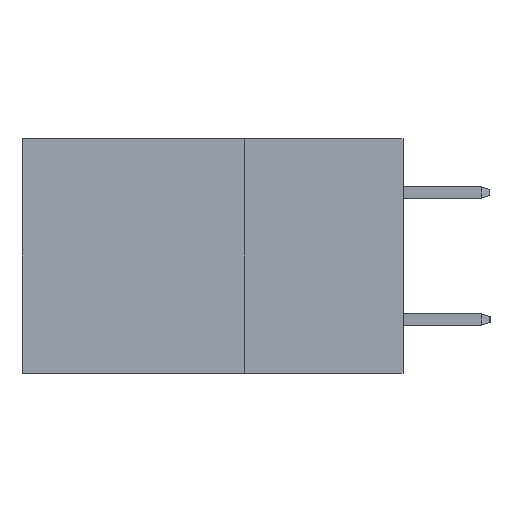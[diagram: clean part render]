
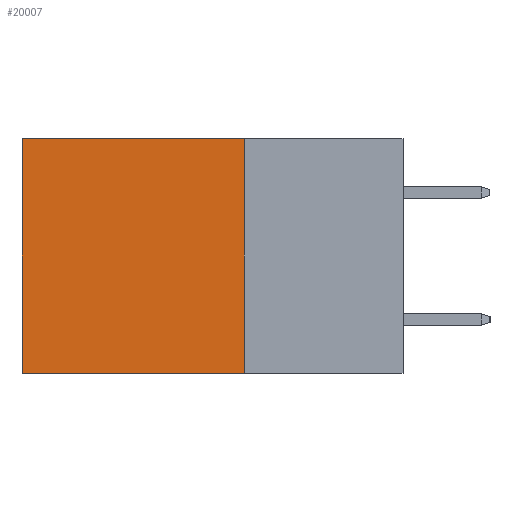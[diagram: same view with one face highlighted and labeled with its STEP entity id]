
A CAD part, left-side view. The second image highlights one B-rep face of the part: STEP entity #20007.
In plain terms, the highlighted planar face has unit normal (-1, 0, 0).
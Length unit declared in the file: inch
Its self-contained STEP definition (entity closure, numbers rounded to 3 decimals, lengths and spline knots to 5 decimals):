
#1389 = ORIENTED_EDGE ( 'NONE', *, *, #18552, .T. ) ;
#2370 = VECTOR ( 'NONE', #10295, 39.37008 ) ;
#5081 = CARTESIAN_POINT ( 'NONE',  ( 0.2875, 0.25, 0. ) ) ;
#5689 = VECTOR ( 'NONE', #16254, 39.37008 ) ;
#5801 = CARTESIAN_POINT ( 'NONE',  ( 0.2875, 0.6, -0.37 ) ) ;
#6368 = VERTEX_POINT ( 'NONE', #16422 ) ;
#6404 = ORIENTED_EDGE ( 'NONE', *, *, #15718, .F. ) ;
#7039 = VECTOR ( 'NONE', #16018, 39.37008 ) ;
#7768 = CARTESIAN_POINT ( 'NONE',  ( 0.2875, 0.25, 0. ) ) ;
#8070 = VERTEX_POINT ( 'NONE', #12647 ) ;
#8123 = PLANE ( 'NONE',  #14566 ) ;
#8311 = CARTESIAN_POINT ( 'NONE',  ( 0.2875, 0.25, -0.37 ) ) ;
#8497 = LINE ( 'NONE', #16744, #8843 ) ;
#8843 = VECTOR ( 'NONE', #18199, 39.37008 ) ;
#9466 = ORIENTED_EDGE ( 'NONE', *, *, #10419, .T. ) ;
#10295 = DIRECTION ( 'NONE',  ( 0., 1., 0. ) ) ;
#10419 = EDGE_CURVE ( 'NONE', #8070, #10884, #11561, .T. ) ;
#10424 = EDGE_CURVE ( 'NONE', #17160, #10884, #13322, .T. ) ;
#10884 = VERTEX_POINT ( 'NONE', #5801 ) ;
#11474 = DIRECTION ( 'NONE',  ( 0., 0., -1. ) ) ;
#11561 = LINE ( 'NONE', #19651, #5689 ) ;
#12615 = FACE_OUTER_BOUND ( 'NONE', #17420, .T. ) ;
#12647 = CARTESIAN_POINT ( 'NONE',  ( 0.2875, 0.6, 0. ) ) ;
#13322 = LINE ( 'NONE', #8311, #2370 ) ;
#13399 = CARTESIAN_POINT ( 'NONE',  ( 0.2875, 0.25, -0.37 ) ) ;
#14237 = LINE ( 'NONE', #7768, #7039 ) ;
#14566 = AXIS2_PLACEMENT_3D ( 'NONE', #5081, #19069, #11474 ) ;
#15238 = ORIENTED_EDGE ( 'NONE', *, *, #10424, .F. ) ;
#15718 = EDGE_CURVE ( 'NONE', #6368, #17160, #14237, .T. ) ;
#16018 = DIRECTION ( 'NONE',  ( 0., 0., -1. ) ) ;
#16254 = DIRECTION ( 'NONE',  ( 0., 0., -1. ) ) ;
#16422 = CARTESIAN_POINT ( 'NONE',  ( 0.2875, 0.25, 0. ) ) ;
#16744 = CARTESIAN_POINT ( 'NONE',  ( 0.2875, 0.25, 0. ) ) ;
#17160 = VERTEX_POINT ( 'NONE', #13399 ) ;
#17420 = EDGE_LOOP ( 'NONE', ( #9466, #15238, #6404, #1389 ) ) ;
#18199 = DIRECTION ( 'NONE',  ( 0., 1., 0. ) ) ;
#18552 = EDGE_CURVE ( 'NONE', #6368, #8070, #8497, .T. ) ;
#19069 = DIRECTION ( 'NONE',  ( 1., 0., 0. ) ) ;
#19651 = CARTESIAN_POINT ( 'NONE',  ( 0.2875, 0.6, 0. ) ) ;
#20007 = ADVANCED_FACE ( 'NONE', ( #12615 ), #8123, .F. ) ;
